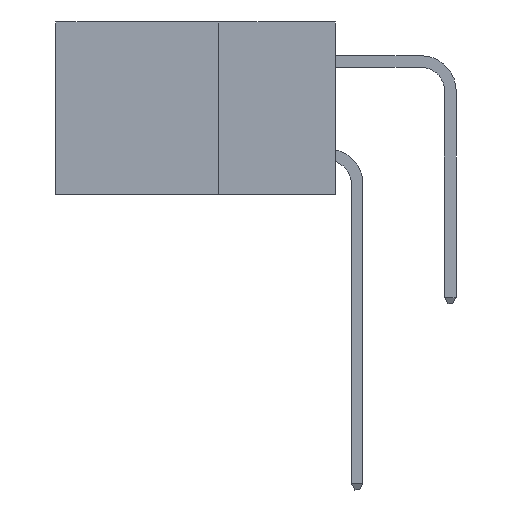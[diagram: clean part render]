
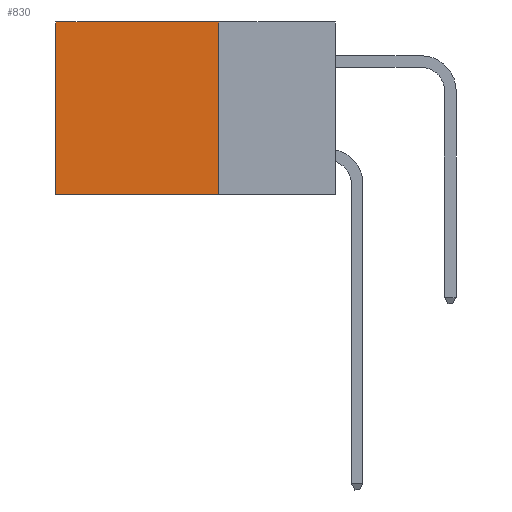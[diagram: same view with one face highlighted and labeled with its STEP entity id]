
A CAD part, left-side view. The second image highlights one B-rep face of the part: STEP entity #830.
In plain terms, the highlighted planar face has unit normal (-1, 0, 0).
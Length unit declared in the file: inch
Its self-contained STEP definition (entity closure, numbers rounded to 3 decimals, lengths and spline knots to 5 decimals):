
#288 = ORIENTED_EDGE ( 'NONE', *, *, #15328, .T. ) ;
#292 = DIRECTION ( 'NONE',  ( 0., 1., 0. ) ) ;
#830 = ADVANCED_FACE ( 'NONE', ( #12640 ), #21267, .F. ) ;
#858 = VERTEX_POINT ( 'NONE', #36693 ) ;
#2889 = VECTOR ( 'NONE', #19440, 39.37008 ) ;
#3435 = ORIENTED_EDGE ( 'NONE', *, *, #12167, .F. ) ;
#3733 = VECTOR ( 'NONE', #25591, 39.37008 ) ;
#4981 = VERTEX_POINT ( 'NONE', #12134 ) ;
#4990 = VECTOR ( 'NONE', #39165, 39.37008 ) ;
#5901 = VERTEX_POINT ( 'NONE', #10075 ) ;
#9104 = DIRECTION ( 'NONE',  ( 1., 0., 0. ) ) ;
#10075 = CARTESIAN_POINT ( 'NONE',  ( 0.2875, 0.25, 0. ) ) ;
#12134 = CARTESIAN_POINT ( 'NONE',  ( 0.2875, 0.6, -0.37 ) ) ;
#12167 = EDGE_CURVE ( 'NONE', #5901, #858, #20078, .T. ) ;
#12640 = FACE_OUTER_BOUND ( 'NONE', #26007, .T. ) ;
#14373 = ORIENTED_EDGE ( 'NONE', *, *, #37883, .T. ) ;
#15019 = CARTESIAN_POINT ( 'NONE',  ( 0.2875, 0.6, 0. ) ) ;
#15328 = EDGE_CURVE ( 'NONE', #17647, #4981, #34536, .T. ) ;
#15908 = EDGE_CURVE ( 'NONE', #858, #4981, #19705, .T. ) ;
#16371 = CARTESIAN_POINT ( 'NONE',  ( 0.2875, 0.6, 0. ) ) ;
#17647 = VERTEX_POINT ( 'NONE', #15019 ) ;
#19440 = DIRECTION ( 'NONE',  ( 0., 0., -1. ) ) ;
#19705 = LINE ( 'NONE', #37092, #34966 ) ;
#20078 = LINE ( 'NONE', #37650, #3733 ) ;
#21267 = PLANE ( 'NONE',  #22648 ) ;
#21274 = LINE ( 'NONE', #36163, #4990 ) ;
#21434 = ORIENTED_EDGE ( 'NONE', *, *, #15908, .F. ) ;
#22648 = AXIS2_PLACEMENT_3D ( 'NONE', #27404, #9104, #30463 ) ;
#25591 = DIRECTION ( 'NONE',  ( 0., 0., -1. ) ) ;
#26007 = EDGE_LOOP ( 'NONE', ( #288, #21434, #3435, #14373 ) ) ;
#27404 = CARTESIAN_POINT ( 'NONE',  ( 0.2875, 0.25, 0. ) ) ;
#30463 = DIRECTION ( 'NONE',  ( 0., 0., -1. ) ) ;
#34536 = LINE ( 'NONE', #16371, #2889 ) ;
#34966 = VECTOR ( 'NONE', #292, 39.37008 ) ;
#36163 = CARTESIAN_POINT ( 'NONE',  ( 0.2875, 0.25, 0. ) ) ;
#36693 = CARTESIAN_POINT ( 'NONE',  ( 0.2875, 0.25, -0.37 ) ) ;
#37092 = CARTESIAN_POINT ( 'NONE',  ( 0.2875, 0.25, -0.37 ) ) ;
#37650 = CARTESIAN_POINT ( 'NONE',  ( 0.2875, 0.25, 0. ) ) ;
#37883 = EDGE_CURVE ( 'NONE', #5901, #17647, #21274, .T. ) ;
#39165 = DIRECTION ( 'NONE',  ( 0., 1., 0. ) ) ;
